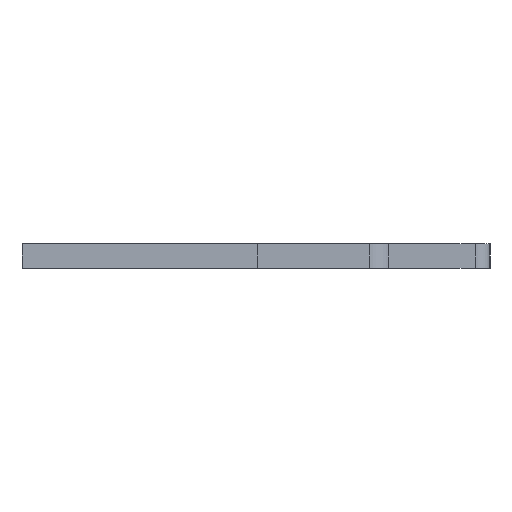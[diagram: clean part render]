
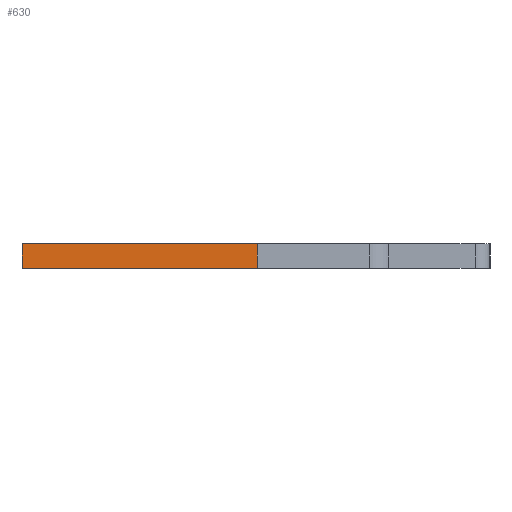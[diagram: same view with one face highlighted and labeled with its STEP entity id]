
A CAD part, left-side view. The second image highlights one B-rep face of the part: STEP entity #630.
In plain terms, the highlighted face is planar.
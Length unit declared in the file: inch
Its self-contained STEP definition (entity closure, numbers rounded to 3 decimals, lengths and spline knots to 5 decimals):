
#64 = LINE ( 'NONE', #1106, #616 ) ;
#91 = VECTOR ( 'NONE', #875, 39.37008 ) ;
#291 = CARTESIAN_POINT ( 'NONE',  ( -0.01, 0.15, -0.04 ) ) ;
#292 = ORIENTED_EDGE ( 'NONE', *, *, #397, .F. ) ;
#360 = EDGE_CURVE ( 'NONE', #1229, #1415, #1619, .T. ) ;
#397 = EDGE_CURVE ( 'NONE', #1415, #968, #853, .T. ) ;
#405 = ORIENTED_EDGE ( 'NONE', *, *, #1652, .T. ) ;
#462 = VECTOR ( 'NONE', #1348, 39.37008 ) ;
#479 = FACE_OUTER_BOUND ( 'NONE', #1628, .T. ) ;
#502 = VERTEX_POINT ( 'NONE', #635 ) ;
#613 = CARTESIAN_POINT ( 'NONE',  ( 0.01, 0.15, -0.04 ) ) ;
#616 = VECTOR ( 'NONE', #1496, 39.37008 ) ;
#630 = ADVANCED_FACE ( 'NONE', ( #479 ), #1244, .F. ) ;
#635 = CARTESIAN_POINT ( 'NONE',  ( -0.01, -0.04, -0.04 ) ) ;
#655 = CARTESIAN_POINT ( 'NONE',  ( 0.01, -0.04, -0.04 ) ) ;
#853 = LINE ( 'NONE', #1765, #462 ) ;
#875 = DIRECTION ( 'NONE',  ( 0., 1., 0. ) ) ;
#968 = VERTEX_POINT ( 'NONE', #1274 ) ;
#985 = LINE ( 'NONE', #291, #1319 ) ;
#1106 = CARTESIAN_POINT ( 'NONE',  ( 0.01, -0.04, -0.04 ) ) ;
#1110 = DIRECTION ( 'NONE',  ( 0., 0., 1. ) ) ;
#1229 = VERTEX_POINT ( 'NONE', #655 ) ;
#1244 = PLANE ( 'NONE',  #1361 ) ;
#1266 = EDGE_CURVE ( 'NONE', #1229, #502, #64, .T. ) ;
#1274 = CARTESIAN_POINT ( 'NONE',  ( -0.01, 0.15, -0.04 ) ) ;
#1319 = VECTOR ( 'NONE', #1581, 39.37008 ) ;
#1348 = DIRECTION ( 'NONE',  ( -1., 0., 0. ) ) ;
#1361 = AXIS2_PLACEMENT_3D ( 'NONE', #1668, #1110, #1511 ) ;
#1396 = ORIENTED_EDGE ( 'NONE', *, *, #360, .F. ) ;
#1415 = VERTEX_POINT ( 'NONE', #613 ) ;
#1496 = DIRECTION ( 'NONE',  ( -1., 0., 0. ) ) ;
#1511 = DIRECTION ( 'NONE',  ( 1., 0., 0. ) ) ;
#1581 = DIRECTION ( 'NONE',  ( 0., 1., 0. ) ) ;
#1583 = ORIENTED_EDGE ( 'NONE', *, *, #1266, .T. ) ;
#1619 = LINE ( 'NONE', #1733, #91 ) ;
#1628 = EDGE_LOOP ( 'NONE', ( #405, #292, #1396, #1583 ) ) ;
#1652 = EDGE_CURVE ( 'NONE', #502, #968, #985, .T. ) ;
#1668 = CARTESIAN_POINT ( 'NONE',  ( 0.01, 0.15, -0.04 ) ) ;
#1733 = CARTESIAN_POINT ( 'NONE',  ( 0.01, 0.15, -0.04 ) ) ;
#1765 = CARTESIAN_POINT ( 'NONE',  ( 0.01, 0.15, -0.04 ) ) ;
